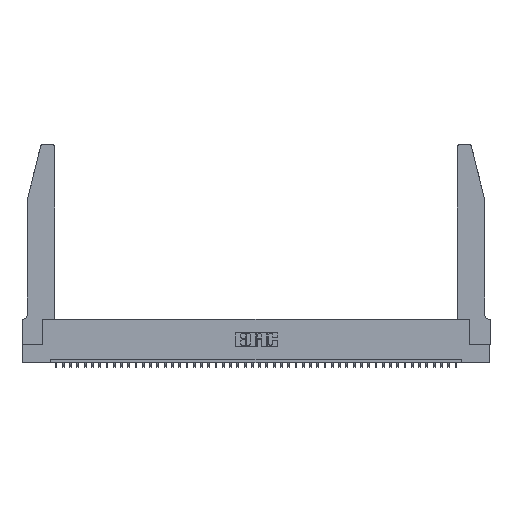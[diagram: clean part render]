
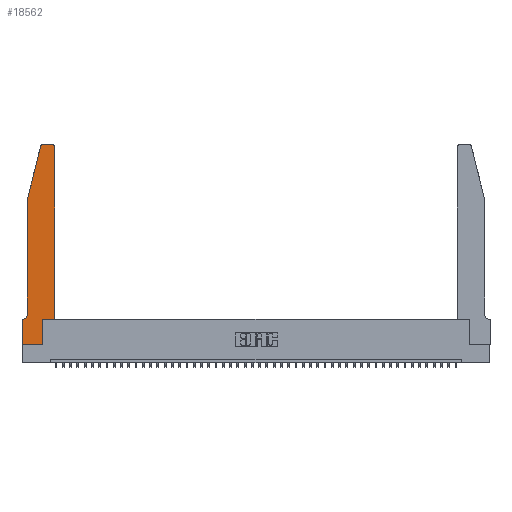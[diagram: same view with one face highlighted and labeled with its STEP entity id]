
A CAD part, top view. The second image highlights one B-rep face of the part: STEP entity #18562.
In plain terms, the highlighted planar face has unit normal (0, 0, 1).
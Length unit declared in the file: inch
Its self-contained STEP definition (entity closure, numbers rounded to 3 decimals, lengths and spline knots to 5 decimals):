
#105 = CARTESIAN_POINT ( 'NONE',  ( 0.284, 2.72, 0.37 ) ) ;
#238 = EDGE_CURVE ( 'NONE', #45053, #21788, #18808, .T. ) ;
#755 = LINE ( 'NONE', #5569, #34482 ) ;
#1466 = CARTESIAN_POINT ( 'NONE',  ( 0.4505, 0.35, 0.37 ) ) ;
#1891 = ORIENTED_EDGE ( 'NONE', *, *, #43944, .T. ) ;
#2357 = LINE ( 'NONE', #22252, #27382 ) ;
#3742 = CARTESIAN_POINT ( 'NONE',  ( 0., 0.35, 0.37 ) ) ;
#3984 = DIRECTION ( 'NONE',  ( -1., 0., 0. ) ) ;
#4554 = CARTESIAN_POINT ( 'NONE',  ( 0.2605, 2.75, 0.37 ) ) ;
#4976 = VERTEX_POINT ( 'NONE', #40466 ) ;
#5569 = CARTESIAN_POINT ( 'NONE',  ( 0.4505, 0.35, 0.37 ) ) ;
#6106 = CARTESIAN_POINT ( 'NONE',  ( 0.2865, 0.35, 0.37 ) ) ;
#6114 = EDGE_CURVE ( 'NONE', #23330, #4976, #755, .T. ) ;
#6316 = EDGE_CURVE ( 'NONE', #20383, #29034, #22030, .T. ) ;
#6355 = AXIS2_PLACEMENT_3D ( 'NONE', #14007, #7450, #41767 ) ;
#7248 = FACE_OUTER_BOUND ( 'NONE', #8933, .T. ) ;
#7269 = DIRECTION ( 'NONE',  ( 1., 0., 0. ) ) ;
#7450 = DIRECTION ( 'NONE',  ( 0., 0., -1. ) ) ;
#7501 = CARTESIAN_POINT ( 'NONE',  ( 0.4205, 2.72, 0.37 ) ) ;
#7533 = AXIS2_PLACEMENT_3D ( 'NONE', #7501, #31768, #31924 ) ;
#7588 = VERTEX_POINT ( 'NONE', #11605 ) ;
#7696 = CIRCLE ( 'NONE', #7533, 0.03 ) ;
#8037 = CARTESIAN_POINT ( 'NONE',  ( 0.0755, 2., 0.37 ) ) ;
#8933 = EDGE_LOOP ( 'NONE', ( #27001, #34779, #21969, #41055, #30847, #33252, #1891, #32973, #26491, #30866, #43946, #28058 ) ) ;
#9500 = EDGE_CURVE ( 'NONE', #7588, #34002, #25712, .T. ) ;
#9944 = EDGE_CURVE ( 'NONE', #12239, #32557, #7696, .T. ) ;
#11605 = CARTESIAN_POINT ( 'NONE',  ( 0.0755, 0.42, 0.37 ) ) ;
#11627 = EDGE_CURVE ( 'NONE', #29034, #7588, #39045, .T. ) ;
#12239 = VERTEX_POINT ( 'NONE', #32763 ) ;
#12263 = CARTESIAN_POINT ( 'NONE',  ( 0., 0.35, 0.37 ) ) ;
#14007 = CARTESIAN_POINT ( 'NONE',  ( 0.0055, 0.42, 0.37 ) ) ;
#14205 = CARTESIAN_POINT ( 'NONE',  ( 0.0055, 0.35, 0.37 ) ) ;
#15640 = DIRECTION ( 'NONE',  ( 0., 1., 0. ) ) ;
#16568 = VECTOR ( 'NONE', #16864, 39.37008 ) ;
#16830 = AXIS2_PLACEMENT_3D ( 'NONE', #105, #44993, #41745 ) ;
#16864 = DIRECTION ( 'NONE',  ( -0.239, -0.971, 0. ) ) ;
#17261 = DIRECTION ( 'NONE',  ( 1., 0., 0. ) ) ;
#18283 = EDGE_CURVE ( 'NONE', #21788, #23330, #2357, .T. ) ;
#18562 = ADVANCED_FACE ( 'NONE', ( #7248 ), #24629, .T. ) ;
#18808 = LINE ( 'NONE', #44455, #26930 ) ;
#19006 = VERTEX_POINT ( 'NONE', #38419 ) ;
#20255 = CARTESIAN_POINT ( 'NONE',  ( 0.0755, 2., 0.37 ) ) ;
#20383 = VERTEX_POINT ( 'NONE', #32809 ) ;
#20663 = VECTOR ( 'NONE', #29496, 39.37008 ) ;
#21788 = VERTEX_POINT ( 'NONE', #38886 ) ;
#21969 = ORIENTED_EDGE ( 'NONE', *, *, #6316, .T. ) ;
#22030 = LINE ( 'NONE', #20255, #16568 ) ;
#22252 = CARTESIAN_POINT ( 'NONE',  ( 0.2865, 0.35, 0.37 ) ) ;
#22802 = VECTOR ( 'NONE', #41069, 39.37008 ) ;
#23078 = EDGE_CURVE ( 'NONE', #32557, #19006, #42663, .T. ) ;
#23330 = VERTEX_POINT ( 'NONE', #6106 ) ;
#23679 = CARTESIAN_POINT ( 'NONE',  ( 0.0755, 2., 0.37 ) ) ;
#24586 = EDGE_CURVE ( 'NONE', #4976, #12239, #33832, .T. ) ;
#24629 = PLANE ( 'NONE',  #38584 ) ;
#25712 = CIRCLE ( 'NONE', #6355, 0.07 ) ;
#26038 = CARTESIAN_POINT ( 'NONE',  ( 0., 0., 0.37 ) ) ;
#26491 = ORIENTED_EDGE ( 'NONE', *, *, #18283, .T. ) ;
#26684 = EDGE_CURVE ( 'NONE', #34002, #38895, #28722, .T. ) ;
#26930 = VECTOR ( 'NONE', #17261, 39.37008 ) ;
#27001 = ORIENTED_EDGE ( 'NONE', *, *, #23078, .T. ) ;
#27382 = VECTOR ( 'NONE', #37058, 39.37008 ) ;
#28058 = ORIENTED_EDGE ( 'NONE', *, *, #9944, .T. ) ;
#28071 = DIRECTION ( 'NONE',  ( 0., 0., 1. ) ) ;
#28551 = VECTOR ( 'NONE', #29641, 39.37008 ) ;
#28722 = LINE ( 'NONE', #34725, #45075 ) ;
#28890 = CARTESIAN_POINT ( 'NONE',  ( 0., 0., 0.37 ) ) ;
#29034 = VERTEX_POINT ( 'NONE', #8037 ) ;
#29496 = DIRECTION ( 'NONE',  ( 0., -1., 0. ) ) ;
#29641 = DIRECTION ( 'NONE',  ( -1., 0., 0. ) ) ;
#29796 = LINE ( 'NONE', #28890, #20663 ) ;
#30535 = VECTOR ( 'NONE', #15640, 39.37008 ) ;
#30847 = ORIENTED_EDGE ( 'NONE', *, *, #9500, .T. ) ;
#30866 = ORIENTED_EDGE ( 'NONE', *, *, #6114, .T. ) ;
#31064 = DIRECTION ( 'NONE',  ( 1., 0., 0. ) ) ;
#31768 = DIRECTION ( 'NONE',  ( 0., 0., 1. ) ) ;
#31924 = DIRECTION ( 'NONE',  ( 1., 0., 0. ) ) ;
#31943 = CARTESIAN_POINT ( 'NONE',  ( 0.4205, 2.75, 0.37 ) ) ;
#32557 = VERTEX_POINT ( 'NONE', #31943 ) ;
#32763 = CARTESIAN_POINT ( 'NONE',  ( 0.4505, 2.72, 0.37 ) ) ;
#32809 = CARTESIAN_POINT ( 'NONE',  ( 0.25487, 2.72718, 0.37 ) ) ;
#32973 = ORIENTED_EDGE ( 'NONE', *, *, #238, .T. ) ;
#33252 = ORIENTED_EDGE ( 'NONE', *, *, #26684, .T. ) ;
#33306 = CIRCLE ( 'NONE', #16830, 0.03 ) ;
#33832 = LINE ( 'NONE', #1466, #30535 ) ;
#34002 = VERTEX_POINT ( 'NONE', #14205 ) ;
#34482 = VECTOR ( 'NONE', #31064, 39.37008 ) ;
#34725 = CARTESIAN_POINT ( 'NONE',  ( 0.0755, 0.35, 0.37 ) ) ;
#34779 = ORIENTED_EDGE ( 'NONE', *, *, #40777, .T. ) ;
#37058 = DIRECTION ( 'NONE',  ( 0., 1., 0. ) ) ;
#38419 = CARTESIAN_POINT ( 'NONE',  ( 0.284, 2.75, 0.37 ) ) ;
#38584 = AXIS2_PLACEMENT_3D ( 'NONE', #3742, #28071, #7269 ) ;
#38886 = CARTESIAN_POINT ( 'NONE',  ( 0.2865, 0., 0.37 ) ) ;
#38895 = VERTEX_POINT ( 'NONE', #12263 ) ;
#39045 = LINE ( 'NONE', #23679, #22802 ) ;
#40466 = CARTESIAN_POINT ( 'NONE',  ( 0.4505, 0.35, 0.37 ) ) ;
#40777 = EDGE_CURVE ( 'NONE', #19006, #20383, #33306, .T. ) ;
#41055 = ORIENTED_EDGE ( 'NONE', *, *, #11627, .T. ) ;
#41069 = DIRECTION ( 'NONE',  ( 0., -1., 0. ) ) ;
#41745 = DIRECTION ( 'NONE',  ( 1., 0., 0. ) ) ;
#41767 = DIRECTION ( 'NONE',  ( -1., 0., 0. ) ) ;
#42663 = LINE ( 'NONE', #4554, #28551 ) ;
#43944 = EDGE_CURVE ( 'NONE', #38895, #45053, #29796, .T. ) ;
#43946 = ORIENTED_EDGE ( 'NONE', *, *, #24586, .T. ) ;
#44455 = CARTESIAN_POINT ( 'NONE',  ( 0., 0., 0.37 ) ) ;
#44993 = DIRECTION ( 'NONE',  ( 0., 0., 1. ) ) ;
#45053 = VERTEX_POINT ( 'NONE', #26038 ) ;
#45075 = VECTOR ( 'NONE', #3984, 39.37008 ) ;
